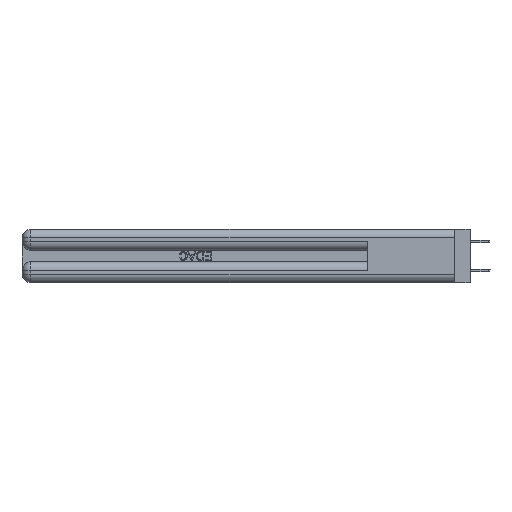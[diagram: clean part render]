
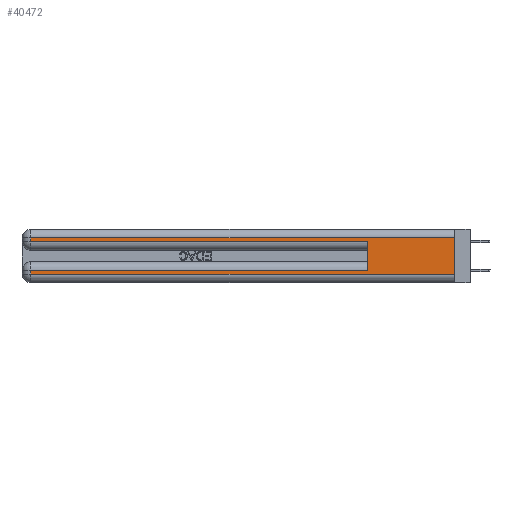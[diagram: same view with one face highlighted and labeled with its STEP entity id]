
A CAD part, left-side view. The second image highlights one B-rep face of the part: STEP entity #40472.
In plain terms, the highlighted planar face has unit normal (-1, 0, 0).
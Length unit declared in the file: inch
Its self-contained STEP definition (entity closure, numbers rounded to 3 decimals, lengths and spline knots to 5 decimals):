
#1193 = ORIENTED_EDGE ( 'NONE', *, *, #4191, .T. ) ;
#1846 = EDGE_CURVE ( 'NONE', #34863, #11911, #36369, .T. ) ;
#2274 = LINE ( 'NONE', #46262, #9329 ) ;
#2450 = DIRECTION ( 'NONE',  ( 0., -1., 0. ) ) ;
#3384 = ORIENTED_EDGE ( 'NONE', *, *, #11877, .T. ) ;
#3706 = LINE ( 'NONE', #10926, #32877 ) ;
#4191 = EDGE_CURVE ( 'NONE', #9510, #22934, #3706, .T. ) ;
#5585 = DIRECTION ( 'NONE',  ( 0., 0., -1. ) ) ;
#5831 = ORIENTED_EDGE ( 'NONE', *, *, #40362, .T. ) ;
#6057 = CARTESIAN_POINT ( 'NONE',  ( 0., 0., 0.37 ) ) ;
#6788 = CARTESIAN_POINT ( 'NONE',  ( 0., 0.6, 0.085 ) ) ;
#7187 = ORIENTED_EDGE ( 'NONE', *, *, #11119, .T. ) ;
#8005 = EDGE_LOOP ( 'NONE', ( #39308, #3384, #25650, #5831, #31252, #41833, #1193, #7187 ) ) ;
#8771 = DIRECTION ( 'NONE',  ( 0., -1., 0. ) ) ;
#9329 = VECTOR ( 'NONE', #31571, 39.37008 ) ;
#9510 = VERTEX_POINT ( 'NONE', #19151 ) ;
#9532 = CARTESIAN_POINT ( 'NONE',  ( 0., 0., 0.31 ) ) ;
#10216 = VECTOR ( 'NONE', #10621, 39.37008 ) ;
#10621 = DIRECTION ( 'NONE',  ( 0., 0., -1. ) ) ;
#10926 = CARTESIAN_POINT ( 'NONE',  ( 0., 2.94, 0.37 ) ) ;
#11100 = VECTOR ( 'NONE', #34166, 39.37008 ) ;
#11119 = EDGE_CURVE ( 'NONE', #22934, #35348, #35127, .T. ) ;
#11877 = EDGE_CURVE ( 'NONE', #16317, #41905, #2274, .T. ) ;
#11911 = VERTEX_POINT ( 'NONE', #18360 ) ;
#12068 = VERTEX_POINT ( 'NONE', #18826 ) ;
#15278 = LINE ( 'NONE', #41685, #15848 ) ;
#15347 = EDGE_CURVE ( 'NONE', #16317, #35348, #28158, .T. ) ;
#15848 = VECTOR ( 'NONE', #8771, 39.37008 ) ;
#16317 = VERTEX_POINT ( 'NONE', #9532 ) ;
#17274 = CARTESIAN_POINT ( 'NONE',  ( 0., 2.94, 0.37 ) ) ;
#18360 = CARTESIAN_POINT ( 'NONE',  ( 0., 0.6, 0.285 ) ) ;
#18826 = CARTESIAN_POINT ( 'NONE',  ( 0., 2.94, 0.285 ) ) ;
#19151 = CARTESIAN_POINT ( 'NONE',  ( 0., 2.94, 0.085 ) ) ;
#21373 = VECTOR ( 'NONE', #24739, 39.37008 ) ;
#22934 = VERTEX_POINT ( 'NONE', #42496 ) ;
#24279 = AXIS2_PLACEMENT_3D ( 'NONE', #6057, #35829, #5585 ) ;
#24739 = DIRECTION ( 'NONE',  ( 0., 0., -1. ) ) ;
#25555 = CARTESIAN_POINT ( 'NONE',  ( 0., 0.6, 0.145 ) ) ;
#25650 = ORIENTED_EDGE ( 'NONE', *, *, #43434, .T. ) ;
#28158 = LINE ( 'NONE', #32220, #10216 ) ;
#28567 = CARTESIAN_POINT ( 'NONE',  ( 0., 0., 0.085 ) ) ;
#29576 = CARTESIAN_POINT ( 'NONE',  ( 0., 2.94, 0.31 ) ) ;
#31252 = ORIENTED_EDGE ( 'NONE', *, *, #1846, .F. ) ;
#31571 = DIRECTION ( 'NONE',  ( 0., 1., 0. ) ) ;
#32149 = LINE ( 'NONE', #28567, #11100 ) ;
#32220 = CARTESIAN_POINT ( 'NONE',  ( 0., 0., 0.37 ) ) ;
#32877 = VECTOR ( 'NONE', #47450, 39.37008 ) ;
#34166 = DIRECTION ( 'NONE',  ( 0., 1., 0. ) ) ;
#34863 = VERTEX_POINT ( 'NONE', #6788 ) ;
#35127 = LINE ( 'NONE', #38976, #40001 ) ;
#35348 = VERTEX_POINT ( 'NONE', #40600 ) ;
#35829 = DIRECTION ( 'NONE',  ( 1., 0., 0. ) ) ;
#35904 = VECTOR ( 'NONE', #43585, 39.37008 ) ;
#36369 = LINE ( 'NONE', #25555, #35904 ) ;
#38192 = EDGE_CURVE ( 'NONE', #34863, #9510, #32149, .T. ) ;
#38497 = PLANE ( 'NONE',  #24279 ) ;
#38681 = LINE ( 'NONE', #17274, #21373 ) ;
#38976 = CARTESIAN_POINT ( 'NONE',  ( 0., 0., 0.06 ) ) ;
#39308 = ORIENTED_EDGE ( 'NONE', *, *, #15347, .F. ) ;
#40001 = VECTOR ( 'NONE', #2450, 39.37008 ) ;
#40362 = EDGE_CURVE ( 'NONE', #12068, #11911, #15278, .T. ) ;
#40472 = ADVANCED_FACE ( 'NONE', ( #42099 ), #38497, .F. ) ;
#40600 = CARTESIAN_POINT ( 'NONE',  ( 0., 0., 0.06 ) ) ;
#41685 = CARTESIAN_POINT ( 'NONE',  ( 0., 0., 0.285 ) ) ;
#41833 = ORIENTED_EDGE ( 'NONE', *, *, #38192, .T. ) ;
#41905 = VERTEX_POINT ( 'NONE', #29576 ) ;
#42099 = FACE_OUTER_BOUND ( 'NONE', #8005, .T. ) ;
#42496 = CARTESIAN_POINT ( 'NONE',  ( 0., 2.94, 0.06 ) ) ;
#43434 = EDGE_CURVE ( 'NONE', #41905, #12068, #38681, .T. ) ;
#43585 = DIRECTION ( 'NONE',  ( 0., 0., 1. ) ) ;
#46262 = CARTESIAN_POINT ( 'NONE',  ( 0., 0., 0.31 ) ) ;
#47450 = DIRECTION ( 'NONE',  ( 0., 0., -1. ) ) ;
